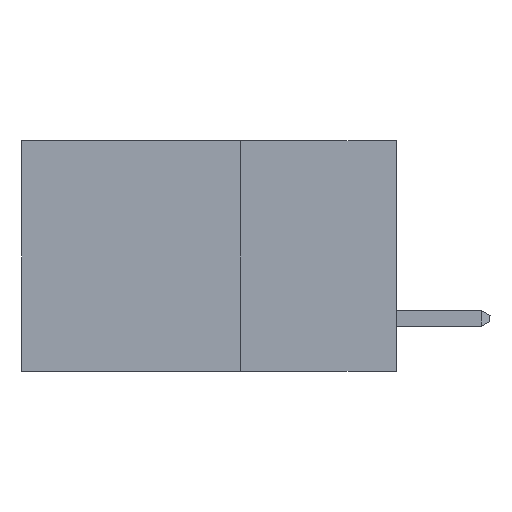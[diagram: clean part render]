
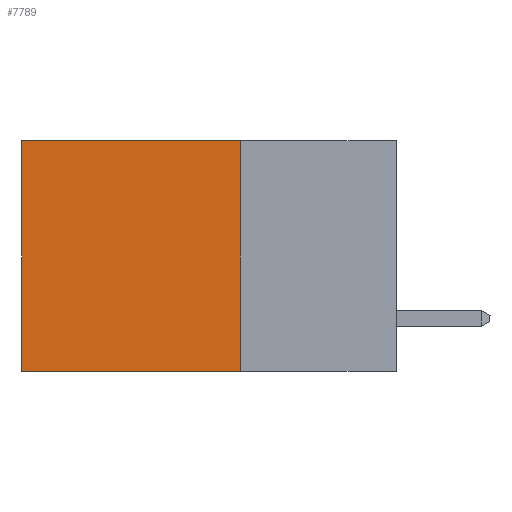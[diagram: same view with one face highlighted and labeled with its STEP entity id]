
A CAD part, left-side view. The second image highlights one B-rep face of the part: STEP entity #7789.
In plain terms, the highlighted planar face has unit normal (-1, 0, 0).
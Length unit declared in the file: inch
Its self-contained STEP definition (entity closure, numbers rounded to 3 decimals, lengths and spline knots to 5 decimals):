
#2311 = DIRECTION ( 'NONE',  ( 0., 0., -1. ) ) ;
#2740 = EDGE_CURVE ( 'NONE', #7011, #18489, #16364, .T. ) ;
#3714 = DIRECTION ( 'NONE',  ( 0., 0., -1. ) ) ;
#4054 = VECTOR ( 'NONE', #2311, 39.37008 ) ;
#4525 = VECTOR ( 'NONE', #6426, 39.37008 ) ;
#4606 = CARTESIAN_POINT ( 'NONE',  ( 0.2615, 0.6, -0.37 ) ) ;
#4621 = CARTESIAN_POINT ( 'NONE',  ( 0.2615, 0.25, -0.37 ) ) ;
#5289 = CARTESIAN_POINT ( 'NONE',  ( 0.2615, 0.6, 0. ) ) ;
#5600 = DIRECTION ( 'NONE',  ( 1., 0., 0. ) ) ;
#5720 = PLANE ( 'NONE',  #24405 ) ;
#6412 = CARTESIAN_POINT ( 'NONE',  ( 0.2615, 0.6, -0.37 ) ) ;
#6426 = DIRECTION ( 'NONE',  ( 0., 1., 0. ) ) ;
#6651 = EDGE_LOOP ( 'NONE', ( #11961, #19740, #18522, #21548 ) ) ;
#7011 = VERTEX_POINT ( 'NONE', #9663 ) ;
#7789 = ADVANCED_FACE ( 'NONE', ( #18034 ), #5720, .F. ) ;
#9663 = CARTESIAN_POINT ( 'NONE',  ( 0.2615, 0.25, 0. ) ) ;
#10501 = LINE ( 'NONE', #4606, #4054 ) ;
#11256 = VECTOR ( 'NONE', #12689, 39.37008 ) ;
#11961 = ORIENTED_EDGE ( 'NONE', *, *, #24103, .T. ) ;
#12299 = LINE ( 'NONE', #24372, #12492 ) ;
#12492 = VECTOR ( 'NONE', #25974, 39.37008 ) ;
#12689 = DIRECTION ( 'NONE',  ( 0., 1., 0. ) ) ;
#12824 = LINE ( 'NONE', #4621, #11256 ) ;
#13096 = CARTESIAN_POINT ( 'NONE',  ( 0.2615, 0.25, -0.37 ) ) ;
#15650 = CARTESIAN_POINT ( 'NONE',  ( 0.2615, 0.25, -0.37 ) ) ;
#16364 = LINE ( 'NONE', #18238, #4525 ) ;
#18034 = FACE_OUTER_BOUND ( 'NONE', #6651, .T. ) ;
#18238 = CARTESIAN_POINT ( 'NONE',  ( 0.2615, 0.25, 0. ) ) ;
#18389 = VERTEX_POINT ( 'NONE', #13096 ) ;
#18489 = VERTEX_POINT ( 'NONE', #5289 ) ;
#18522 = ORIENTED_EDGE ( 'NONE', *, *, #23224, .F. ) ;
#19120 = VERTEX_POINT ( 'NONE', #6412 ) ;
#19740 = ORIENTED_EDGE ( 'NONE', *, *, #23457, .F. ) ;
#21548 = ORIENTED_EDGE ( 'NONE', *, *, #2740, .T. ) ;
#23224 = EDGE_CURVE ( 'NONE', #7011, #18389, #12299, .T. ) ;
#23457 = EDGE_CURVE ( 'NONE', #18389, #19120, #12824, .T. ) ;
#24103 = EDGE_CURVE ( 'NONE', #18489, #19120, #10501, .T. ) ;
#24372 = CARTESIAN_POINT ( 'NONE',  ( 0.2615, 0.25, -0.37 ) ) ;
#24405 = AXIS2_PLACEMENT_3D ( 'NONE', #15650, #5600, #3714 ) ;
#25974 = DIRECTION ( 'NONE',  ( 0., 0., -1. ) ) ;
